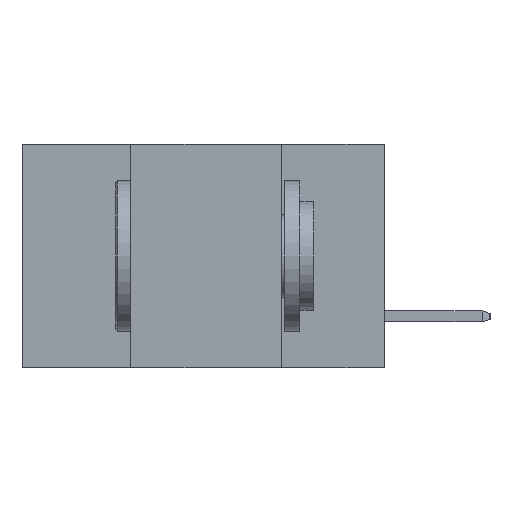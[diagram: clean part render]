
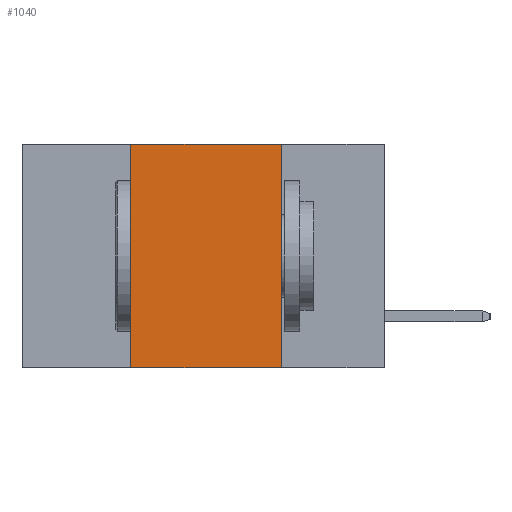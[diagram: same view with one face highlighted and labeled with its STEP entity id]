
A CAD part, left-side view. The second image highlights one B-rep face of the part: STEP entity #1040.
In plain terms, the highlighted planar face has unit normal (-1, 0, 0).
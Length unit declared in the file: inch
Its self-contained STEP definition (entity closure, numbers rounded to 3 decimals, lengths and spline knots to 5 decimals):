
#391 = EDGE_CURVE ( 'NONE', #14792, #7332, #15749, .T. ) ;
#708 = CARTESIAN_POINT ( 'NONE',  ( 0., 0.42, 0. ) ) ;
#1040 = ADVANCED_FACE ( 'NONE', ( #18829 ), #10749, .F. ) ;
#1515 = VECTOR ( 'NONE', #12716, 39.37008 ) ;
#2542 = ORIENTED_EDGE ( 'NONE', *, *, #6379, .F. ) ;
#3206 = EDGE_LOOP ( 'NONE', ( #2542, #14454, #18282, #18718 ) ) ;
#3393 = VECTOR ( 'NONE', #11771, 39.37008 ) ;
#3883 = VECTOR ( 'NONE', #8226, 39.37008 ) ;
#4364 = LINE ( 'NONE', #4901, #3883 ) ;
#4901 = CARTESIAN_POINT ( 'NONE',  ( 0., 0.6, -0.37 ) ) ;
#5681 = AXIS2_PLACEMENT_3D ( 'NONE', #7890, #5816, #6303 ) ;
#5714 = EDGE_CURVE ( 'NONE', #14360, #14184, #4364, .T. ) ;
#5816 = DIRECTION ( 'NONE',  ( 1., 0., 0. ) ) ;
#5931 = CARTESIAN_POINT ( 'NONE',  ( 0., 0.6, 0. ) ) ;
#6303 = DIRECTION ( 'NONE',  ( 0., 0., -1. ) ) ;
#6379 = EDGE_CURVE ( 'NONE', #7332, #14184, #12060, .T. ) ;
#7270 = CARTESIAN_POINT ( 'NONE',  ( 0., 0.17, 0. ) ) ;
#7291 = DIRECTION ( 'NONE',  ( 0., 0., -1. ) ) ;
#7332 = VERTEX_POINT ( 'NONE', #13301 ) ;
#7494 = CARTESIAN_POINT ( 'NONE',  ( 0., 0.42, 0. ) ) ;
#7890 = CARTESIAN_POINT ( 'NONE',  ( 0., 0.6, 0. ) ) ;
#8226 = DIRECTION ( 'NONE',  ( 0., -1., 0. ) ) ;
#10749 = PLANE ( 'NONE',  #5681 ) ;
#11771 = DIRECTION ( 'NONE',  ( 0., -1., 0. ) ) ;
#12060 = LINE ( 'NONE', #7270, #15513 ) ;
#12716 = DIRECTION ( 'NONE',  ( 0., 0., 1. ) ) ;
#13301 = CARTESIAN_POINT ( 'NONE',  ( 0., 0.17, 0. ) ) ;
#13477 = LINE ( 'NONE', #708, #1515 ) ;
#13794 = CARTESIAN_POINT ( 'NONE',  ( 0., 0.42, -0.37 ) ) ;
#14184 = VERTEX_POINT ( 'NONE', #17699 ) ;
#14360 = VERTEX_POINT ( 'NONE', #13794 ) ;
#14454 = ORIENTED_EDGE ( 'NONE', *, *, #391, .F. ) ;
#14792 = VERTEX_POINT ( 'NONE', #7494 ) ;
#15513 = VECTOR ( 'NONE', #7291, 39.37008 ) ;
#15749 = LINE ( 'NONE', #5931, #3393 ) ;
#16993 = EDGE_CURVE ( 'NONE', #14360, #14792, #13477, .T. ) ;
#17699 = CARTESIAN_POINT ( 'NONE',  ( 0., 0.17, -0.37 ) ) ;
#18282 = ORIENTED_EDGE ( 'NONE', *, *, #16993, .F. ) ;
#18718 = ORIENTED_EDGE ( 'NONE', *, *, #5714, .T. ) ;
#18829 = FACE_OUTER_BOUND ( 'NONE', #3206, .T. ) ;
